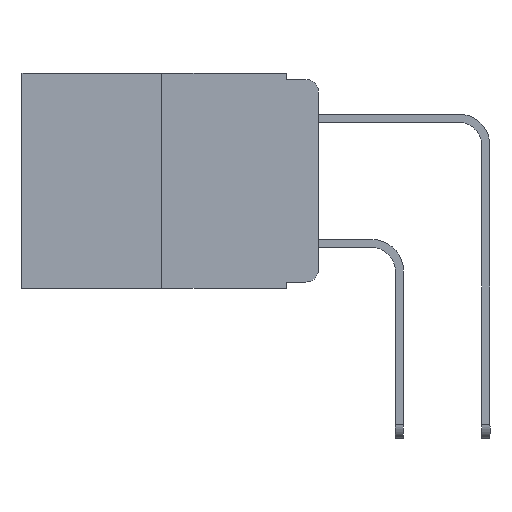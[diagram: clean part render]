
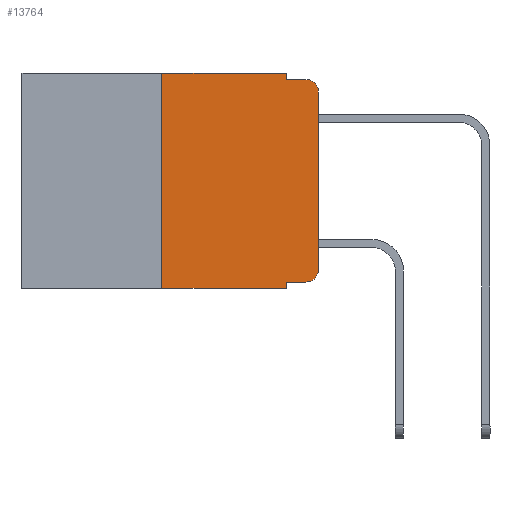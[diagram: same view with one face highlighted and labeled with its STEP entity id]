
A CAD part, left-side view. The second image highlights one B-rep face of the part: STEP entity #13764.
In plain terms, the highlighted planar face has unit normal (-1, 0, 0).
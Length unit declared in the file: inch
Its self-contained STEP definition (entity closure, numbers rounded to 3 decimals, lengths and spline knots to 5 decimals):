
#144 = FACE_OUTER_BOUND ( 'NONE', #16815, .T. ) ;
#294 = VERTEX_POINT ( 'NONE', #16448 ) ;
#781 = EDGE_CURVE ( 'NONE', #14398, #13409, #6704, .T. ) ;
#956 = VECTOR ( 'NONE', #13272, 39.37008 ) ;
#993 = LINE ( 'NONE', #18897, #8397 ) ;
#1111 = DIRECTION ( 'NONE',  ( 0., -1., 0. ) ) ;
#1270 = EDGE_CURVE ( 'NONE', #12459, #1773, #11884, .T. ) ;
#1456 = CARTESIAN_POINT ( 'NONE',  ( 0., 0.473, 0. ) ) ;
#1557 = EDGE_CURVE ( 'NONE', #1773, #5389, #6960, .T. ) ;
#1559 = CARTESIAN_POINT ( 'NONE',  ( 0., 0.02, -0.313 ) ) ;
#1589 = CARTESIAN_POINT ( 'NONE',  ( 0., 0.051, -0.01 ) ) ;
#1598 = DIRECTION ( 'NONE',  ( 0., 0., 1. ) ) ;
#1773 = VERTEX_POINT ( 'NONE', #1589 ) ;
#2045 = EDGE_CURVE ( 'NONE', #13409, #13097, #6735, .T. ) ;
#2379 = ORIENTED_EDGE ( 'NONE', *, *, #17110, .F. ) ;
#2566 = LINE ( 'NONE', #3840, #9952 ) ;
#2923 = DIRECTION ( 'NONE',  ( -1., 0., 0. ) ) ;
#3193 = LINE ( 'NONE', #10536, #956 ) ;
#3282 = CARTESIAN_POINT ( 'NONE',  ( 0., 0.02, -0.01 ) ) ;
#3739 = CARTESIAN_POINT ( 'NONE',  ( 0., 0.051, -0.01 ) ) ;
#3840 = CARTESIAN_POINT ( 'NONE',  ( 0., 0.051, -0.333 ) ) ;
#4101 = DIRECTION ( 'NONE',  ( 0., 0., -1. ) ) ;
#4145 = DIRECTION ( 'NONE',  ( -1., 0., 0. ) ) ;
#4501 = VECTOR ( 'NONE', #7156, 39.37008 ) ;
#4524 = LINE ( 'NONE', #4708, #9183 ) ;
#4528 = DIRECTION ( 'NONE',  ( 1., 0., 0. ) ) ;
#4667 = VERTEX_POINT ( 'NONE', #8311 ) ;
#4708 = CARTESIAN_POINT ( 'NONE',  ( 0., 0.25, 0. ) ) ;
#5389 = VERTEX_POINT ( 'NONE', #3282 ) ;
#5599 = CARTESIAN_POINT ( 'NONE',  ( 0., 0.02, -0.03 ) ) ;
#5699 = CARTESIAN_POINT ( 'NONE',  ( 0., 0.051, -0.343 ) ) ;
#5711 = AXIS2_PLACEMENT_3D ( 'NONE', #5599, #4145, #12837 ) ;
#5822 = VECTOR ( 'NONE', #18991, 39.37008 ) ;
#6150 = CARTESIAN_POINT ( 'NONE',  ( 0., 0., -0.03 ) ) ;
#6454 = VERTEX_POINT ( 'NONE', #17495 ) ;
#6525 = EDGE_CURVE ( 'NONE', #6454, #17003, #3193, .T. ) ;
#6704 = CIRCLE ( 'NONE', #9231, 0.02 ) ;
#6735 = LINE ( 'NONE', #7032, #5822 ) ;
#6960 = LINE ( 'NONE', #3739, #4501 ) ;
#7032 = CARTESIAN_POINT ( 'NONE',  ( 0., 0., 0. ) ) ;
#7156 = DIRECTION ( 'NONE',  ( 0., -1., 0. ) ) ;
#7186 = ORIENTED_EDGE ( 'NONE', *, *, #10708, .T. ) ;
#7208 = VECTOR ( 'NONE', #10082, 39.37008 ) ;
#7576 = CARTESIAN_POINT ( 'NONE',  ( 0., 0., -0.313 ) ) ;
#8311 = CARTESIAN_POINT ( 'NONE',  ( 0., 0.051, -0.333 ) ) ;
#8397 = VECTOR ( 'NONE', #11453, 39.37008 ) ;
#8866 = ORIENTED_EDGE ( 'NONE', *, *, #17013, .T. ) ;
#9183 = VECTOR ( 'NONE', #1598, 39.37008 ) ;
#9231 = AXIS2_PLACEMENT_3D ( 'NONE', #1559, #2923, #4101 ) ;
#9746 = VECTOR ( 'NONE', #17940, 39.37008 ) ;
#9952 = VECTOR ( 'NONE', #1111, 39.37008 ) ;
#10082 = DIRECTION ( 'NONE',  ( 0., -1., 0. ) ) ;
#10416 = CARTESIAN_POINT ( 'NONE',  ( 0., 0.051, 0. ) ) ;
#10536 = CARTESIAN_POINT ( 'NONE',  ( 0., 0.473, -0.343 ) ) ;
#10708 = EDGE_CURVE ( 'NONE', #4667, #14398, #2566, .T. ) ;
#11082 = ORIENTED_EDGE ( 'NONE', *, *, #2045, .T. ) ;
#11132 = EDGE_CURVE ( 'NONE', #4667, #17003, #993, .T. ) ;
#11453 = DIRECTION ( 'NONE',  ( 0., 0., -1. ) ) ;
#11884 = LINE ( 'NONE', #13526, #9746 ) ;
#12060 = CARTESIAN_POINT ( 'NONE',  ( 0., 0.473, 0. ) ) ;
#12459 = VERTEX_POINT ( 'NONE', #10416 ) ;
#12519 = ORIENTED_EDGE ( 'NONE', *, *, #1270, .F. ) ;
#12603 = CARTESIAN_POINT ( 'NONE',  ( 0., 0.02, -0.333 ) ) ;
#12837 = DIRECTION ( 'NONE',  ( 0., 0., -1. ) ) ;
#13097 = VERTEX_POINT ( 'NONE', #6150 ) ;
#13272 = DIRECTION ( 'NONE',  ( 0., -1., 0. ) ) ;
#13409 = VERTEX_POINT ( 'NONE', #7576 ) ;
#13526 = CARTESIAN_POINT ( 'NONE',  ( 0., 0.051, 0. ) ) ;
#13764 = ADVANCED_FACE ( 'NONE', ( #144 ), #17652, .F. ) ;
#13789 = AXIS2_PLACEMENT_3D ( 'NONE', #12060, #4528, #16286 ) ;
#14398 = VERTEX_POINT ( 'NONE', #12603 ) ;
#14509 = ORIENTED_EDGE ( 'NONE', *, *, #1557, .F. ) ;
#14511 = EDGE_CURVE ( 'NONE', #294, #12459, #14576, .T. ) ;
#14576 = LINE ( 'NONE', #1456, #7208 ) ;
#15803 = ORIENTED_EDGE ( 'NONE', *, *, #11132, .F. ) ;
#16286 = DIRECTION ( 'NONE',  ( 0., 0., -1. ) ) ;
#16448 = CARTESIAN_POINT ( 'NONE',  ( 0., 0.25, 0. ) ) ;
#16577 = ORIENTED_EDGE ( 'NONE', *, *, #781, .T. ) ;
#16815 = EDGE_LOOP ( 'NONE', ( #11082, #8866, #14509, #12519, #17821, #2379, #17784, #15803, #7186, #16577 ) ) ;
#17003 = VERTEX_POINT ( 'NONE', #5699 ) ;
#17013 = EDGE_CURVE ( 'NONE', #13097, #5389, #17284, .T. ) ;
#17110 = EDGE_CURVE ( 'NONE', #6454, #294, #4524, .T. ) ;
#17284 = CIRCLE ( 'NONE', #5711, 0.02 ) ;
#17495 = CARTESIAN_POINT ( 'NONE',  ( 0., 0.25, -0.343 ) ) ;
#17652 = PLANE ( 'NONE',  #13789 ) ;
#17784 = ORIENTED_EDGE ( 'NONE', *, *, #6525, .T. ) ;
#17821 = ORIENTED_EDGE ( 'NONE', *, *, #14511, .F. ) ;
#17940 = DIRECTION ( 'NONE',  ( 0., 0., -1. ) ) ;
#18897 = CARTESIAN_POINT ( 'NONE',  ( 0., 0.051, 0. ) ) ;
#18991 = DIRECTION ( 'NONE',  ( 0., 0., 1. ) ) ;
